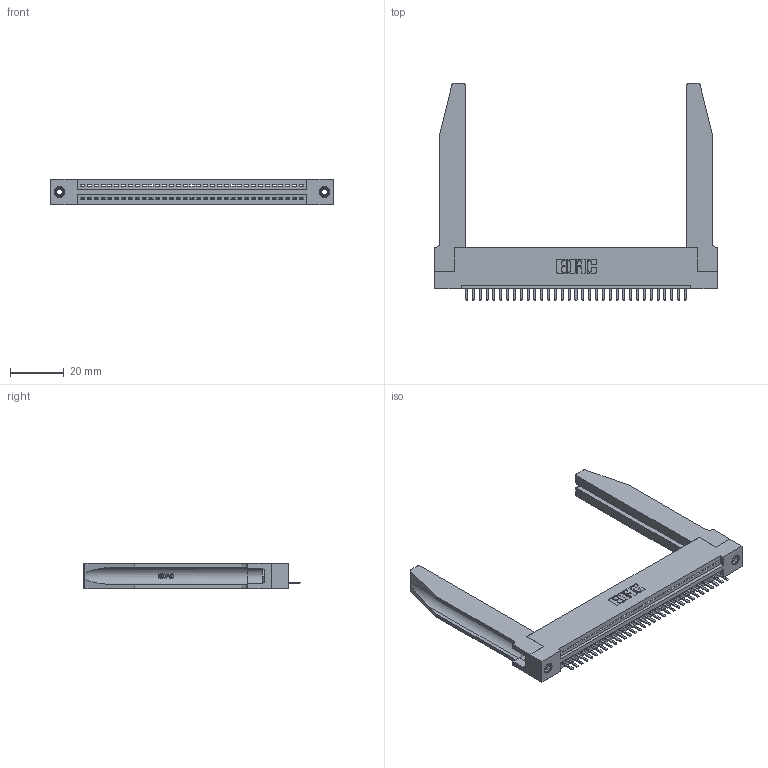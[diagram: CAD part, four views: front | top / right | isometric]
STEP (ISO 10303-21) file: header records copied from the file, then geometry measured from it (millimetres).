
FILE_DESCRIPTION (( 'STEP AP203' ), '1' );
FILE_NAME ('395-033-520-178.STEP', '2019-10-19T15:10:55', ( '' ), ( '' ), 'SwSTEP 2.0', 'SolidWorks 2016', '' );
FILE_SCHEMA (( 'CONFIG_CONTROL_DESIGN' ));
Length unit declared in the file: inch
Products named in the file (5): 345-292-001_345-293-120; 395-033-520-178; 345-220-078_345-220-078; 345 Part_Flush Mounting Lugs - 0.156 Dia-TH; 345-250-001_345-250-001-102
Assembly tree (38 placements, depth 2):
  395-033-520-178
    345 Part_Flush Mounting Lugs - 0.156 Dia-TH
    345-292-001_345-293-120  x33
    345-250-001_345-250-001-102  x2
    345-220-078_345-220-078  x2
Bounding box: 105.05 x 80.64 x 9.4 mm (x, y, z)
Volume: 17580 mm3; surface area: 19448.7 mm2
Topology: 38 solids, 38 shells, 2406 faces, 7021 edges, 4582 vertices
Faces by surface type: plane 1608, cylinder 746, bspline 36, cone 12, torus 4
Entity records: 30902 total; most frequent: CARTESIAN_POINT 6262, ORIENTED_EDGE 5114, DIRECTION 4477, EDGE_CURVE 2557, VECTOR 2195, LINE 2195, VERTEX_POINT 1696, AXIS2_PLACEMENT_3D 1141
